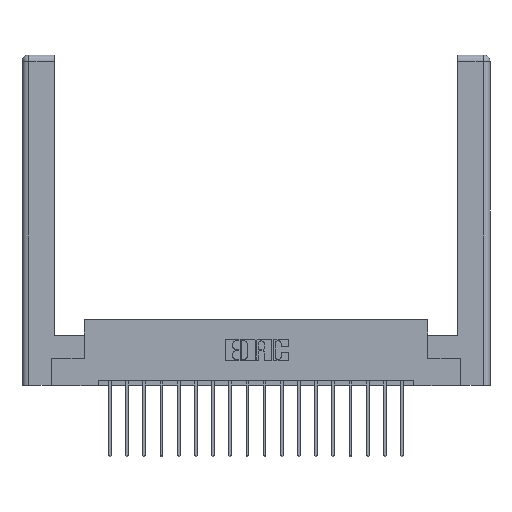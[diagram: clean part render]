
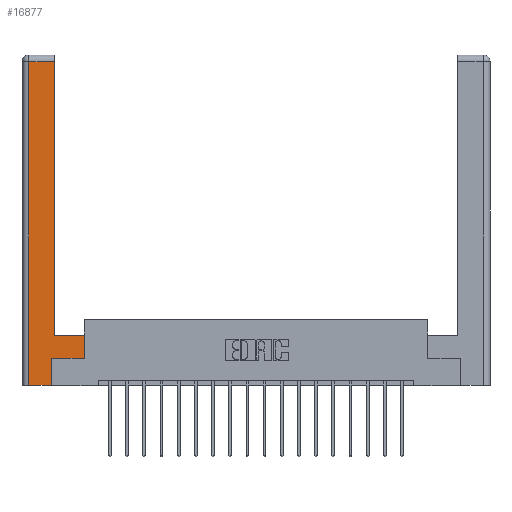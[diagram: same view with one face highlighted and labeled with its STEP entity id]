
A CAD part, top view. The second image highlights one B-rep face of the part: STEP entity #16877.
In plain terms, the highlighted planar face has unit normal (0, 0, 1).
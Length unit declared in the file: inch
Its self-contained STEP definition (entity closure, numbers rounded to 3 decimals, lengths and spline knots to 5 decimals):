
#94 = DIRECTION ( 'NONE',  ( 0., 1., 0. ) ) ;
#132 = VECTOR ( 'NONE', #444, 39.37008 ) ;
#444 = DIRECTION ( 'NONE',  ( 1., 0., 0. ) ) ;
#739 = VECTOR ( 'NONE', #94, 39.37008 ) ;
#1345 = CARTESIAN_POINT ( 'NONE',  ( 0.0615, 0., 0. ) ) ;
#1746 = EDGE_LOOP ( 'NONE', ( #9113, #4706, #19430, #5328, #2370, #15198, #6919, #4613 ) ) ;
#1803 = CARTESIAN_POINT ( 'NONE',  ( 0.265, 0.245, 0. ) ) ;
#2059 = VECTOR ( 'NONE', #3850, 39.37008 ) ;
#2370 = ORIENTED_EDGE ( 'NONE', *, *, #15758, .T. ) ;
#2666 = CARTESIAN_POINT ( 'NONE',  ( 0.295, 2.94, 0. ) ) ;
#2891 = VECTOR ( 'NONE', #8917, 39.37008 ) ;
#2976 = CARTESIAN_POINT ( 'NONE',  ( 0.565, 0.245, 0. ) ) ;
#3850 = DIRECTION ( 'NONE',  ( 0., -1., 0. ) ) ;
#3887 = CARTESIAN_POINT ( 'NONE',  ( 0.565, 0.245, 0. ) ) ;
#3949 = DIRECTION ( 'NONE',  ( 1., 0., 0. ) ) ;
#4613 = ORIENTED_EDGE ( 'NONE', *, *, #6305, .T. ) ;
#4706 = ORIENTED_EDGE ( 'NONE', *, *, #18996, .T. ) ;
#5328 = ORIENTED_EDGE ( 'NONE', *, *, #18554, .T. ) ;
#6238 = CARTESIAN_POINT ( 'NONE',  ( 0.565, 0.45, 0. ) ) ;
#6282 = VECTOR ( 'NONE', #15836, 39.37008 ) ;
#6305 = EDGE_CURVE ( 'NONE', #18964, #6538, #18443, .T. ) ;
#6310 = CARTESIAN_POINT ( 'NONE',  ( 0.0615, 2.94, 0. ) ) ;
#6538 = VERTEX_POINT ( 'NONE', #11352 ) ;
#6837 = PLANE ( 'NONE',  #15309 ) ;
#6919 = ORIENTED_EDGE ( 'NONE', *, *, #15670, .T. ) ;
#7139 = CARTESIAN_POINT ( 'NONE',  ( 0.565, 0.45, 0. ) ) ;
#7300 = VECTOR ( 'NONE', #16890, 39.37008 ) ;
#7406 = LINE ( 'NONE', #7139, #2891 ) ;
#7801 = VECTOR ( 'NONE', #3949, 39.37008 ) ;
#7884 = DIRECTION ( 'NONE',  ( -1., 0., 0. ) ) ;
#8190 = LINE ( 'NONE', #17322, #6282 ) ;
#8350 = DIRECTION ( 'NONE',  ( 0., 0., -1. ) ) ;
#8364 = LINE ( 'NONE', #1803, #739 ) ;
#8917 = DIRECTION ( 'NONE',  ( 0., 1., 0. ) ) ;
#8987 = VERTEX_POINT ( 'NONE', #19669 ) ;
#9113 = ORIENTED_EDGE ( 'NONE', *, *, #14286, .T. ) ;
#10574 = VERTEX_POINT ( 'NONE', #2976 ) ;
#11352 = CARTESIAN_POINT ( 'NONE',  ( 0.295, 0.45, 0. ) ) ;
#11530 = EDGE_CURVE ( 'NONE', #13722, #10574, #11829, .T. ) ;
#11829 = LINE ( 'NONE', #3887, #7801 ) ;
#12281 = CARTESIAN_POINT ( 'NONE',  ( 0.295, 0.45, 0. ) ) ;
#12523 = EDGE_CURVE ( 'NONE', #17662, #12834, #13906, .T. ) ;
#12585 = CARTESIAN_POINT ( 'NONE',  ( 0.265, 0.245, 0. ) ) ;
#12834 = VERTEX_POINT ( 'NONE', #1345 ) ;
#13722 = VERTEX_POINT ( 'NONE', #12585 ) ;
#13906 = LINE ( 'NONE', #18559, #2059 ) ;
#14243 = DIRECTION ( 'NONE',  ( -1., 0., 0. ) ) ;
#14286 = EDGE_CURVE ( 'NONE', #6538, #16836, #8190, .T. ) ;
#14418 = LINE ( 'NONE', #6310, #14893 ) ;
#14893 = VECTOR ( 'NONE', #7884, 39.37008 ) ;
#15198 = ORIENTED_EDGE ( 'NONE', *, *, #11530, .T. ) ;
#15309 = AXIS2_PLACEMENT_3D ( 'NONE', #15837, #8350, #14243 ) ;
#15670 = EDGE_CURVE ( 'NONE', #10574, #18964, #7406, .T. ) ;
#15758 = EDGE_CURVE ( 'NONE', #8987, #13722, #8364, .T. ) ;
#15836 = DIRECTION ( 'NONE',  ( 0., 1., 0. ) ) ;
#15837 = CARTESIAN_POINT ( 'NONE',  ( 0., 0., 0. ) ) ;
#16039 = CARTESIAN_POINT ( 'NONE',  ( 0.0615, 2.94, 0. ) ) ;
#16099 = LINE ( 'NONE', #18684, #132 ) ;
#16836 = VERTEX_POINT ( 'NONE', #2666 ) ;
#16877 = ADVANCED_FACE ( 'NONE', ( #18062 ), #6837, .F. ) ;
#16890 = DIRECTION ( 'NONE',  ( -1., 0., 0. ) ) ;
#17322 = CARTESIAN_POINT ( 'NONE',  ( 0.295, 3., 0. ) ) ;
#17662 = VERTEX_POINT ( 'NONE', #16039 ) ;
#18062 = FACE_OUTER_BOUND ( 'NONE', #1746, .T. ) ;
#18443 = LINE ( 'NONE', #12281, #7300 ) ;
#18554 = EDGE_CURVE ( 'NONE', #12834, #8987, #16099, .T. ) ;
#18559 = CARTESIAN_POINT ( 'NONE',  ( 0.0615, 0., 0. ) ) ;
#18684 = CARTESIAN_POINT ( 'NONE',  ( 0.265, 0., 0. ) ) ;
#18964 = VERTEX_POINT ( 'NONE', #6238 ) ;
#18996 = EDGE_CURVE ( 'NONE', #16836, #17662, #14418, .T. ) ;
#19430 = ORIENTED_EDGE ( 'NONE', *, *, #12523, .T. ) ;
#19669 = CARTESIAN_POINT ( 'NONE',  ( 0.265, 0., 0. ) ) ;
